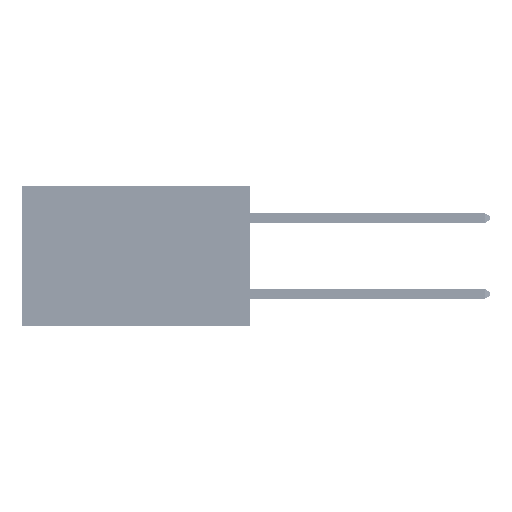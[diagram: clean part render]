
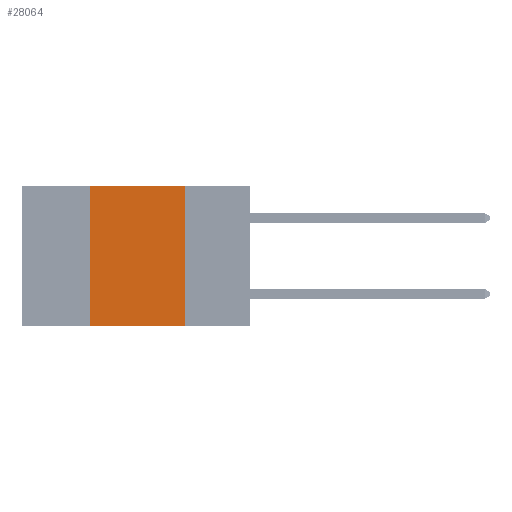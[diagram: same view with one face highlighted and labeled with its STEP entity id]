
A CAD part, left-side view. The second image highlights one B-rep face of the part: STEP entity #28064.
In plain terms, the highlighted planar face has unit normal (-1, 0, 0).
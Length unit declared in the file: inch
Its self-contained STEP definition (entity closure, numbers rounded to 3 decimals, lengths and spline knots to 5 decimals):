
#919 = VECTOR ( 'NONE', #35573, 39.37008 ) ;
#3548 = DIRECTION ( 'NONE',  ( 0., -1., 0. ) ) ;
#4030 = CARTESIAN_POINT ( 'NONE',  ( 0., 0.42, 0. ) ) ;
#4342 = EDGE_CURVE ( 'NONE', #4868, #16444, #22504, .T. ) ;
#4868 = VERTEX_POINT ( 'NONE', #48345 ) ;
#7356 = ORIENTED_EDGE ( 'NONE', *, *, #4342, .F. ) ;
#8092 = ORIENTED_EDGE ( 'NONE', *, *, #28706, .T. ) ;
#11522 = LINE ( 'NONE', #40025, #47420 ) ;
#11914 = VECTOR ( 'NONE', #24607, 39.37008 ) ;
#13104 = CARTESIAN_POINT ( 'NONE',  ( 0., 0.17, 0. ) ) ;
#16444 = VERTEX_POINT ( 'NONE', #36321 ) ;
#16711 = DIRECTION ( 'NONE',  ( 0., -1., 0. ) ) ;
#22504 = LINE ( 'NONE', #13104, #11914 ) ;
#23309 = PLANE ( 'NONE',  #28536 ) ;
#23655 = DIRECTION ( 'NONE',  ( 1., 0., 0. ) ) ;
#24607 = DIRECTION ( 'NONE',  ( 0., 0., -1. ) ) ;
#25132 = VECTOR ( 'NONE', #3548, 39.37008 ) ;
#25174 = EDGE_CURVE ( 'NONE', #47757, #4868, #11522, .T. ) ;
#27428 = EDGE_CURVE ( 'NONE', #39258, #47757, #48036, .T. ) ;
#28064 = ADVANCED_FACE ( 'NONE', ( #45547 ), #23309, .F. ) ;
#28536 = AXIS2_PLACEMENT_3D ( 'NONE', #38798, #23655, #34825 ) ;
#28706 = EDGE_CURVE ( 'NONE', #39258, #16444, #34979, .T. ) ;
#29782 = EDGE_LOOP ( 'NONE', ( #7356, #34055, #45759, #8092 ) ) ;
#34055 = ORIENTED_EDGE ( 'NONE', *, *, #25174, .F. ) ;
#34825 = DIRECTION ( 'NONE',  ( 0., 0., -1. ) ) ;
#34979 = LINE ( 'NONE', #47039, #25132 ) ;
#35573 = DIRECTION ( 'NONE',  ( 0., 0., 1. ) ) ;
#36321 = CARTESIAN_POINT ( 'NONE',  ( 0., 0.17, -0.37 ) ) ;
#38798 = CARTESIAN_POINT ( 'NONE',  ( 0., 0.6, 0. ) ) ;
#39258 = VERTEX_POINT ( 'NONE', #42747 ) ;
#40025 = CARTESIAN_POINT ( 'NONE',  ( 0., 0.6, 0. ) ) ;
#42747 = CARTESIAN_POINT ( 'NONE',  ( 0., 0.42, -0.37 ) ) ;
#45547 = FACE_OUTER_BOUND ( 'NONE', #29782, .T. ) ;
#45759 = ORIENTED_EDGE ( 'NONE', *, *, #27428, .F. ) ;
#47039 = CARTESIAN_POINT ( 'NONE',  ( 0., 0.6, -0.37 ) ) ;
#47420 = VECTOR ( 'NONE', #16711, 39.37008 ) ;
#47757 = VERTEX_POINT ( 'NONE', #50416 ) ;
#48036 = LINE ( 'NONE', #4030, #919 ) ;
#48345 = CARTESIAN_POINT ( 'NONE',  ( 0., 0.17, 0. ) ) ;
#50416 = CARTESIAN_POINT ( 'NONE',  ( 0., 0.42, 0. ) ) ;
